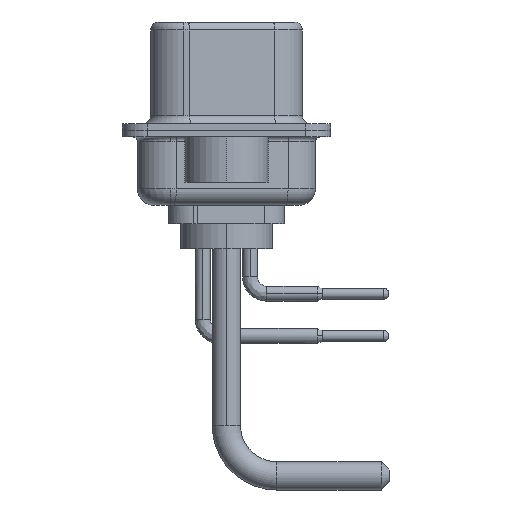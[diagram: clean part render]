
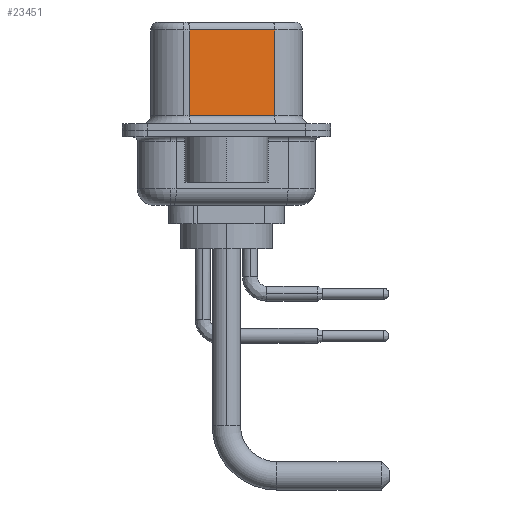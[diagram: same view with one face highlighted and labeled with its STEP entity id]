
A CAD part, left-side view. The second image highlights one B-rep face of the part: STEP entity #23451.
In plain terms, the highlighted planar face has unit normal (-0.985, -0.174, 0).
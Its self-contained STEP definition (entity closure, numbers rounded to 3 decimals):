
#305 = EDGE_LOOP ( 'NONE', ( #4153, #1553, #14895, #2149 ) ) ;
#943 = CARTESIAN_POINT ( 'NONE',  ( 4.58, -2.897, 6.52 ) ) ;
#1088 = VECTOR ( 'NONE', #5955, 1000. ) ;
#1553 = ORIENTED_EDGE ( 'NONE', *, *, #13079, .T. ) ;
#1568 = CARTESIAN_POINT ( 'NONE',  ( 4.58, -2.897, 0.9 ) ) ;
#1990 = VERTEX_POINT ( 'NONE', #13957 ) ;
#2099 = DIRECTION ( 'NONE',  ( 0.174, -0.985, 0. ) ) ;
#2145 = EDGE_CURVE ( 'NONE', #1990, #14445, #20331, .T. ) ;
#2149 = ORIENTED_EDGE ( 'NONE', *, *, #11299, .T. ) ;
#2599 = CARTESIAN_POINT ( 'NONE',  ( 4.58, -2.897, 0.9 ) ) ;
#2821 = DIRECTION ( 'NONE',  ( -0.174, 0.985, 0. ) ) ;
#4153 = ORIENTED_EDGE ( 'NONE', *, *, #12862, .F. ) ;
#4301 = CARTESIAN_POINT ( 'NONE',  ( 4.58, -2.897, 6.02 ) ) ;
#4586 = LINE ( 'NONE', #23428, #23786 ) ;
#5599 = VECTOR ( 'NONE', #23326, 1000. ) ;
#5871 = VERTEX_POINT ( 'NONE', #4301 ) ;
#5955 = DIRECTION ( 'NONE',  ( 0., 0., -1. ) ) ;
#6090 = CARTESIAN_POINT ( 'NONE',  ( 3.68, 2.203, 6.52 ) ) ;
#6788 = LINE ( 'NONE', #943, #5599 ) ;
#9815 = VERTEX_POINT ( 'NONE', #2599 ) ;
#11299 = EDGE_CURVE ( 'NONE', #14445, #9815, #16205, .T. ) ;
#11362 = AXIS2_PLACEMENT_3D ( 'NONE', #24956, #18836, #22792 ) ;
#11965 = FACE_OUTER_BOUND ( 'NONE', #305, .T. ) ;
#12613 = PLANE ( 'NONE',  #11362 ) ;
#12862 = EDGE_CURVE ( 'NONE', #5871, #9815, #6788, .T. ) ;
#13079 = EDGE_CURVE ( 'NONE', #5871, #1990, #4586, .T. ) ;
#13957 = CARTESIAN_POINT ( 'NONE',  ( 3.68, 2.203, 6.02 ) ) ;
#14445 = VERTEX_POINT ( 'NONE', #17358 ) ;
#14895 = ORIENTED_EDGE ( 'NONE', *, *, #2145, .T. ) ;
#16205 = LINE ( 'NONE', #1568, #18133 ) ;
#17358 = CARTESIAN_POINT ( 'NONE',  ( 3.68, 2.203, 0.9 ) ) ;
#18133 = VECTOR ( 'NONE', #2099, 1000. ) ;
#18836 = DIRECTION ( 'NONE',  ( 0.985, 0.174, 0. ) ) ;
#20331 = LINE ( 'NONE', #6090, #1088 ) ;
#22792 = DIRECTION ( 'NONE',  ( -0.174, 0.985, 0. ) ) ;
#23326 = DIRECTION ( 'NONE',  ( 0., 0., -1. ) ) ;
#23428 = CARTESIAN_POINT ( 'NONE',  ( 4.58, -2.897, 6.02 ) ) ;
#23451 = ADVANCED_FACE ( 'NONE', ( #11965 ), #12613, .F. ) ;
#23786 = VECTOR ( 'NONE', #2821, 1000. ) ;
#24956 = CARTESIAN_POINT ( 'NONE',  ( 4.58, -2.897, 6.52 ) ) ;
